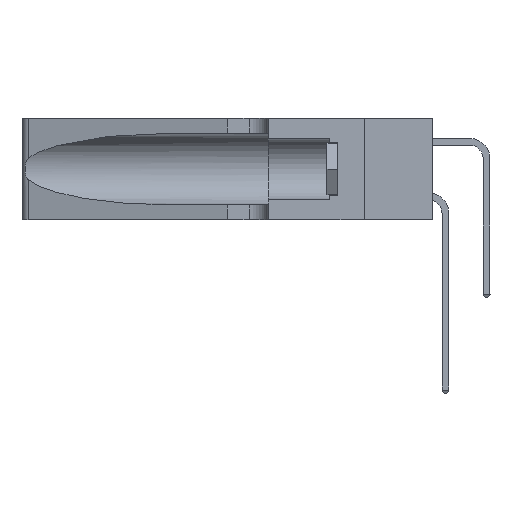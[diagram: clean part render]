
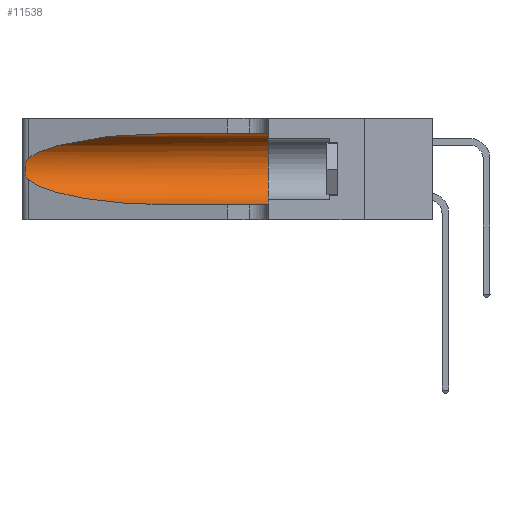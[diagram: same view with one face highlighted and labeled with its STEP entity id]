
A CAD part, left-side view. The second image highlights one B-rep face of the part: STEP entity #11538.
In plain terms, the highlighted cylindrical face has radius 3.308 mm (diameter 6.617 mm), a partial arc.
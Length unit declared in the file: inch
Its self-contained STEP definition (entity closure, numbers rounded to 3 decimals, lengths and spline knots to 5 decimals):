
#84 = AXIS2_PLACEMENT_3D ( 'NONE', #23430, #8853, #25901 ) ;
#232 = CARTESIAN_POINT ( 'NONE',  ( 0.1305, 0.72297, 0.05475 ) ) ;
#1423 = ORIENTED_EDGE ( 'NONE', *, *, #14984, .T. ) ;
#1930 = EDGE_LOOP ( 'NONE', ( #15291, #14954, #1423, #20752, #24042, #16430 ) ) ;
#2812 = EDGE_CURVE ( 'NONE', #11361, #23541, #28054, .T. ) ;
#3734 = CARTESIAN_POINT ( 'NONE',  ( 0.25787, 1.23484, 0.2124 ) ) ;
#5389 = EDGE_CURVE ( 'NONE', #23541, #7152, #28868, .T. ) ;
#5585 = FACE_OUTER_BOUND ( 'NONE', #1930, .T. ) ;
#6148 = CARTESIAN_POINT ( 'NONE',  ( 0.26018, 1.23835, 0.19895 ) ) ;
#7152 = VERTEX_POINT ( 'NONE', #10072 ) ;
#7603 = VERTEX_POINT ( 'NONE', #31207 ) ;
#8155 = CARTESIAN_POINT ( 'NONE',  ( 0.1305, 0.72297, 0.31525 ) ) ;
#8205 = DIRECTION ( 'NONE',  ( 0., -1., 0. ) ) ;
#8615 = CARTESIAN_POINT ( 'NONE',  ( 0.26075, 1.23896, 0.178 ) ) ;
#8853 = DIRECTION ( 'NONE',  ( 0., 1., 0. ) ) ;
#10072 = CARTESIAN_POINT ( 'NONE',  ( 0.1305, 0.35, 0.05475 ) ) ;
#10647 = CARTESIAN_POINT ( 'NONE',  ( 0.18966, 0.96281, 0.31525 ) ) ;
#11119 = CARTESIAN_POINT ( 'NONE',  ( 0.25856, 1.23593, 0.16098 ) ) ;
#11361 = VERTEX_POINT ( 'NONE', #16381 ) ;
#11538 = ADVANCED_FACE ( 'NONE', ( #5585 ), #17844, .F. ) ;
#12481 = CARTESIAN_POINT ( 'NONE',  ( 0.2373, 1.15595, 0.08982 ) ) ;
#12513 = VERTEX_POINT ( 'NONE', #26401 ) ;
#12709 = DIRECTION ( 'NONE',  ( 0., -1., 0. ) ) ;
#13128 = CARTESIAN_POINT ( 'NONE',  ( 0.2373, 1.15595, 0.28018 ) ) ;
#13492 = CARTESIAN_POINT ( 'NONE',  ( 0.25555, 1.22994, 0.2215 ) ) ;
#13583 = CARTESIAN_POINT ( 'NONE',  ( 0.25639, 1.23186, 0.15144 ) ) ;
#13685 = EDGE_CURVE ( 'NONE', #21324, #7603, #25976, .T. ) ;
#14939 = CARTESIAN_POINT ( 'NONE',  ( 0.18966, 0.96281, 0.05475 ) ) ;
#14954 = ORIENTED_EDGE ( 'NONE', *, *, #13685, .T. ) ;
#14984 = EDGE_CURVE ( 'NONE', #7603, #12513, #19724, .T. ) ;
#15291 = ORIENTED_EDGE ( 'NONE', *, *, #20935, .T. ) ;
#16025 = CARTESIAN_POINT ( 'NONE',  ( 0.25487, 1.22718, 0.14631 ) ) ;
#16381 = CARTESIAN_POINT ( 'NONE',  ( 0.1305, 0.72297, 0.31525 ) ) ;
#16430 = ORIENTED_EDGE ( 'NONE', *, *, #2812, .F. ) ;
#17844 = CYLINDRICAL_SURFACE ( 'NONE', #28636, 0.13025 ) ;
#17936 = CARTESIAN_POINT ( 'NONE',  ( 0.1305, 1.61858, 0.185 ) ) ;
#18355 = CARTESIAN_POINT ( 'NONE',  ( 0.25639, 1.23184, 0.21858 ) ) ;
#18797 = LINE ( 'NONE', #27260, #25219 ) ;
#19724 =( BOUNDED_CURVE ( )  B_SPLINE_CURVE ( 3, ( #29503, #12481, #14939, #232 ),
 .UNSPECIFIED., .F., .T. ) 
 B_SPLINE_CURVE_WITH_KNOTS ( ( 4, 4 ),
 ( 3.44316, 4.71239 ),
 .UNSPECIFIED. ) 
 CURVE ( )  GEOMETRIC_REPRESENTATION_ITEM ( )  RATIONAL_B_SPLINE_CURVE ( ( 1., 0.87, 0.87, 1. ) ) 
 REPRESENTATION_ITEM ( '' )  );
#20752 = ORIENTED_EDGE ( 'NONE', *, *, #20816, .T. ) ;
#20786 = CARTESIAN_POINT ( 'NONE',  ( 0.25854, 1.2359, 0.20912 ) ) ;
#20791 = CARTESIAN_POINT ( 'NONE',  ( 0.1305, 1.61858, 0.31525 ) ) ;
#20816 = EDGE_CURVE ( 'NONE', #12513, #7152, #18797, .T. ) ;
#20935 = EDGE_CURVE ( 'NONE', #11361, #21324, #24073, .T. ) ;
#21324 = VERTEX_POINT ( 'NONE', #21894 ) ;
#21566 = VECTOR ( 'NONE', #25662, 39.37008 ) ;
#21894 = CARTESIAN_POINT ( 'NONE',  ( 0.25487, 1.22718, 0.22369 ) ) ;
#23209 = CARTESIAN_POINT ( 'NONE',  ( 0.26075, 1.23896, 0.19203 ) ) ;
#23430 = CARTESIAN_POINT ( 'NONE',  ( 0.1305, 0.35, 0.185 ) ) ;
#23541 = VERTEX_POINT ( 'NONE', #27996 ) ;
#24042 = ORIENTED_EDGE ( 'NONE', *, *, #5389, .F. ) ;
#24073 =( BOUNDED_CURVE ( )  B_SPLINE_CURVE ( 3, ( #8155, #10647, #13128, #30130 ),
 .UNSPECIFIED., .F., .F. ) 
 B_SPLINE_CURVE_WITH_KNOTS ( ( 4, 4 ),
 ( 1.5708, 2.84003 ),
 .UNSPECIFIED. ) 
 CURVE ( )  GEOMETRIC_REPRESENTATION_ITEM ( )  RATIONAL_B_SPLINE_CURVE ( ( 1., 0.87, 0.87, 1. ) ) 
 REPRESENTATION_ITEM ( '' )  );
#25219 = VECTOR ( 'NONE', #12709, 39.37008 ) ;
#25246 = DIRECTION ( 'NONE',  ( 0., 0., -1. ) ) ;
#25657 = CARTESIAN_POINT ( 'NONE',  ( 0.26017, 1.23833, 0.17102 ) ) ;
#25662 = DIRECTION ( 'NONE',  ( 0., -1., 0. ) ) ;
#25901 = DIRECTION ( 'NONE',  ( 0., 0., 1. ) ) ;
#25976 = B_SPLINE_CURVE_WITH_KNOTS ( 'NONE', 3,
 ( #30474, #13492, #18355, #3734, #20786, #6148, #23209, #8615, #25657, #11119, #28138, #13583, #30583, #16025 ),
 .UNSPECIFIED., .F., .F.,
 ( 4, 2, 2, 2, 2, 2, 4 ),
 ( 0., 0.00027, 0.00053, 0.00107, 0.0016, 0.00187, 0.00214 ),
 .UNSPECIFIED. ) ;
#26401 = CARTESIAN_POINT ( 'NONE',  ( 0.1305, 0.72297, 0.05475 ) ) ;
#27260 = CARTESIAN_POINT ( 'NONE',  ( 0.1305, 1.61858, 0.05475 ) ) ;
#27996 = CARTESIAN_POINT ( 'NONE',  ( 0.1305, 0.35, 0.31525 ) ) ;
#28054 = LINE ( 'NONE', #20791, #21566 ) ;
#28138 = CARTESIAN_POINT ( 'NONE',  ( 0.25789, 1.23486, 0.15765 ) ) ;
#28636 = AXIS2_PLACEMENT_3D ( 'NONE', #17936, #8205, #25246 ) ;
#28868 = CIRCLE ( 'NONE', #84, 0.13025 ) ;
#29503 = CARTESIAN_POINT ( 'NONE',  ( 0.25487, 1.22718, 0.14631 ) ) ;
#30130 = CARTESIAN_POINT ( 'NONE',  ( 0.25487, 1.22718, 0.22369 ) ) ;
#30474 = CARTESIAN_POINT ( 'NONE',  ( 0.25487, 1.22718, 0.22369 ) ) ;
#30583 = CARTESIAN_POINT ( 'NONE',  ( 0.25555, 1.22993, 0.14849 ) ) ;
#31207 = CARTESIAN_POINT ( 'NONE',  ( 0.25487, 1.22718, 0.14631 ) ) ;
